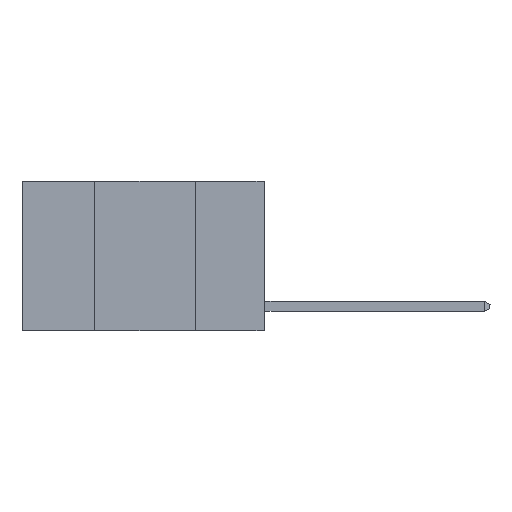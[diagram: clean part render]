
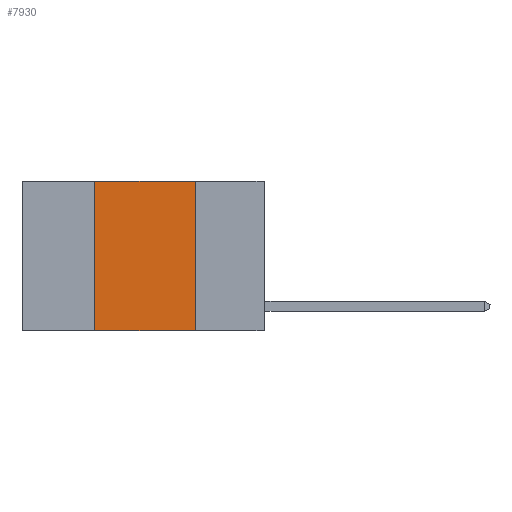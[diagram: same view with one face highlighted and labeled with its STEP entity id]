
A CAD part, left-side view. The second image highlights one B-rep face of the part: STEP entity #7930.
In plain terms, the highlighted planar face has unit normal (-1, 0, 0).
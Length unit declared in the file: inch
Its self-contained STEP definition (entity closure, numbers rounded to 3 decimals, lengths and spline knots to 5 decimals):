
#465 = AXIS2_PLACEMENT_3D ( 'NONE', #471, #1365, #7309 ) ;
#471 = CARTESIAN_POINT ( 'NONE',  ( 0., 0.6, 0. ) ) ;
#1365 = DIRECTION ( 'NONE',  ( 1., 0., 0. ) ) ;
#2084 = VECTOR ( 'NONE', #2220, 39.37008 ) ;
#2195 = VERTEX_POINT ( 'NONE', #7436 ) ;
#2216 = CARTESIAN_POINT ( 'NONE',  ( 0., 0.6, 0. ) ) ;
#2220 = DIRECTION ( 'NONE',  ( 0., 0., -1. ) ) ;
#2274 = EDGE_CURVE ( 'NONE', #9878, #6789, #6074, .T. ) ;
#2439 = ORIENTED_EDGE ( 'NONE', *, *, #2274, .F. ) ;
#2487 = DIRECTION ( 'NONE',  ( 0., 0., 1. ) ) ;
#2521 = LINE ( 'NONE', #2216, #6749 ) ;
#3439 = EDGE_CURVE ( 'NONE', #9878, #2195, #7872, .T. ) ;
#3549 = DIRECTION ( 'NONE',  ( 0., -1., 0. ) ) ;
#4030 = CARTESIAN_POINT ( 'NONE',  ( 0., 0.17, 0. ) ) ;
#4453 = ORIENTED_EDGE ( 'NONE', *, *, #7251, .F. ) ;
#5653 = VECTOR ( 'NONE', #3549, 39.37008 ) ;
#6074 = LINE ( 'NONE', #7546, #8026 ) ;
#6146 = ORIENTED_EDGE ( 'NONE', *, *, #3439, .T. ) ;
#6447 = DIRECTION ( 'NONE',  ( 0., -1., 0. ) ) ;
#6642 = CARTESIAN_POINT ( 'NONE',  ( 0., 0.42, 0. ) ) ;
#6749 = VECTOR ( 'NONE', #6447, 39.37008 ) ;
#6789 = VERTEX_POINT ( 'NONE', #6642 ) ;
#6901 = CARTESIAN_POINT ( 'NONE',  ( 0., 0.6, -0.37 ) ) ;
#7251 = EDGE_CURVE ( 'NONE', #6789, #7305, #2521, .T. ) ;
#7289 = CARTESIAN_POINT ( 'NONE',  ( 0., 0.17, 0. ) ) ;
#7305 = VERTEX_POINT ( 'NONE', #4030 ) ;
#7309 = DIRECTION ( 'NONE',  ( 0., 0., -1. ) ) ;
#7436 = CARTESIAN_POINT ( 'NONE',  ( 0., 0.17, -0.37 ) ) ;
#7546 = CARTESIAN_POINT ( 'NONE',  ( 0., 0.42, 0. ) ) ;
#7872 = LINE ( 'NONE', #6901, #5653 ) ;
#7930 = ADVANCED_FACE ( 'NONE', ( #9324 ), #10553, .F. ) ;
#8026 = VECTOR ( 'NONE', #2487, 39.37008 ) ;
#8559 = LINE ( 'NONE', #7289, #2084 ) ;
#8568 = CARTESIAN_POINT ( 'NONE',  ( 0., 0.42, -0.37 ) ) ;
#8653 = EDGE_LOOP ( 'NONE', ( #10062, #4453, #2439, #6146 ) ) ;
#9324 = FACE_OUTER_BOUND ( 'NONE', #8653, .T. ) ;
#9878 = VERTEX_POINT ( 'NONE', #8568 ) ;
#10062 = ORIENTED_EDGE ( 'NONE', *, *, #10114, .F. ) ;
#10114 = EDGE_CURVE ( 'NONE', #7305, #2195, #8559, .T. ) ;
#10553 = PLANE ( 'NONE',  #465 ) ;
